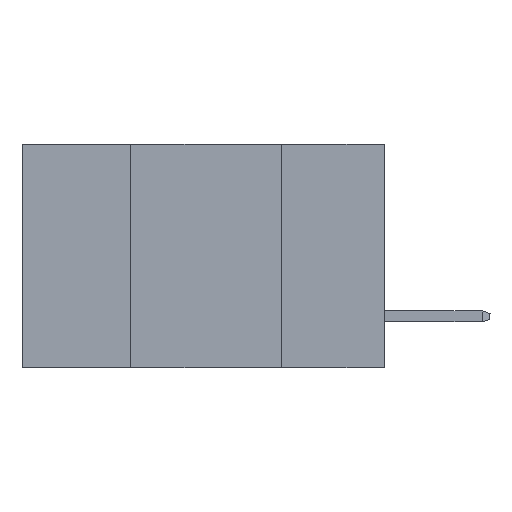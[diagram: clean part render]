
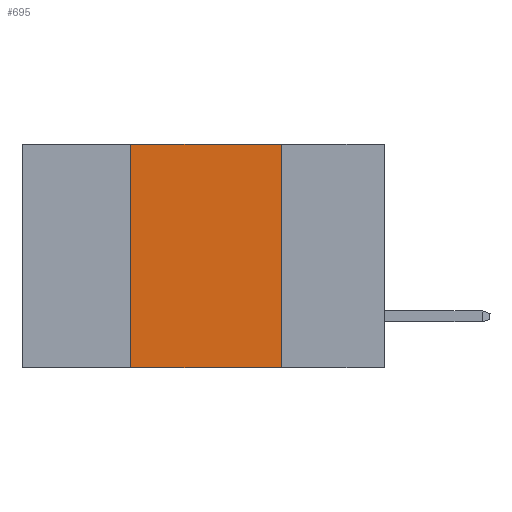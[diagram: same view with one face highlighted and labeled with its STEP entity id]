
A CAD part, left-side view. The second image highlights one B-rep face of the part: STEP entity #695.
In plain terms, the highlighted planar face has unit normal (-1, 0, 0).
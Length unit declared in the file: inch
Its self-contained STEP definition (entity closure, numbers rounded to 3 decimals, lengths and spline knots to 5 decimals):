
#136 = PLANE ( 'NONE',  #22513 ) ;
#246 = CARTESIAN_POINT ( 'NONE',  ( 0., 0.42, 0. ) ) ;
#695 = ADVANCED_FACE ( 'NONE', ( #24335 ), #136, .F. ) ;
#1103 = CARTESIAN_POINT ( 'NONE',  ( 0., 0.6, -0.37 ) ) ;
#1348 = VERTEX_POINT ( 'NONE', #1534 ) ;
#1412 = EDGE_CURVE ( 'NONE', #1348, #1831, #13835, .T. ) ;
#1534 = CARTESIAN_POINT ( 'NONE',  ( 0., 0.17, 0. ) ) ;
#1831 = VERTEX_POINT ( 'NONE', #11574 ) ;
#1857 = DIRECTION ( 'NONE',  ( 0., 0., -1. ) ) ;
#3777 = DIRECTION ( 'NONE',  ( 0., 0., -1. ) ) ;
#5413 = CARTESIAN_POINT ( 'NONE',  ( 0., 0.42, -0.37 ) ) ;
#5815 = EDGE_CURVE ( 'NONE', #9336, #1831, #11531, .T. ) ;
#7131 = VECTOR ( 'NONE', #23160, 39.37008 ) ;
#8890 = EDGE_CURVE ( 'NONE', #13344, #1348, #17119, .T. ) ;
#9169 = DIRECTION ( 'NONE',  ( 0., -1., 0. ) ) ;
#9336 = VERTEX_POINT ( 'NONE', #9755 ) ;
#9449 = VECTOR ( 'NONE', #3777, 39.37008 ) ;
#9755 = CARTESIAN_POINT ( 'NONE',  ( 0., 0.42, -0.37 ) ) ;
#9783 = DIRECTION ( 'NONE',  ( 0., -1., 0. ) ) ;
#10766 = ORIENTED_EDGE ( 'NONE', *, *, #5815, .T. ) ;
#10886 = ORIENTED_EDGE ( 'NONE', *, *, #8890, .F. ) ;
#11531 = LINE ( 'NONE', #1103, #15353 ) ;
#11574 = CARTESIAN_POINT ( 'NONE',  ( 0., 0.17, -0.37 ) ) ;
#12629 = ORIENTED_EDGE ( 'NONE', *, *, #22483, .F. ) ;
#13344 = VERTEX_POINT ( 'NONE', #246 ) ;
#13835 = LINE ( 'NONE', #16219, #9449 ) ;
#15148 = CARTESIAN_POINT ( 'NONE',  ( 0., 0.6, 0. ) ) ;
#15353 = VECTOR ( 'NONE', #9169, 39.37008 ) ;
#15964 = VECTOR ( 'NONE', #9783, 39.37008 ) ;
#16146 = DIRECTION ( 'NONE',  ( 1., 0., 0. ) ) ;
#16219 = CARTESIAN_POINT ( 'NONE',  ( 0., 0.17, -0.37 ) ) ;
#16737 = ORIENTED_EDGE ( 'NONE', *, *, #1412, .F. ) ;
#17119 = LINE ( 'NONE', #15148, #15964 ) ;
#21179 = LINE ( 'NONE', #5413, #7131 ) ;
#21692 = EDGE_LOOP ( 'NONE', ( #16737, #10886, #12629, #10766 ) ) ;
#22483 = EDGE_CURVE ( 'NONE', #9336, #13344, #21179, .T. ) ;
#22513 = AXIS2_PLACEMENT_3D ( 'NONE', #24457, #16146, #1857 ) ;
#23160 = DIRECTION ( 'NONE',  ( 0., 0., 1. ) ) ;
#24335 = FACE_OUTER_BOUND ( 'NONE', #21692, .T. ) ;
#24457 = CARTESIAN_POINT ( 'NONE',  ( 0., 0.6, 0. ) ) ;
